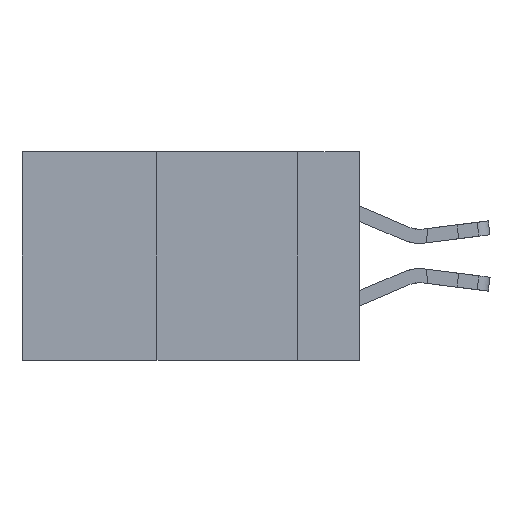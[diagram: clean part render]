
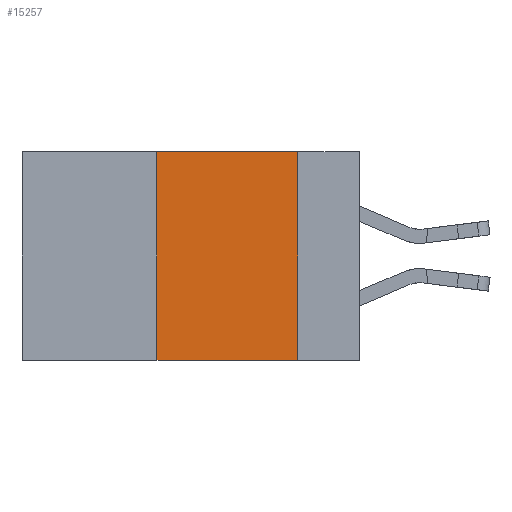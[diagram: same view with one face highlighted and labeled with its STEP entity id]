
A CAD part, left-side view. The second image highlights one B-rep face of the part: STEP entity #15257.
In plain terms, the highlighted planar face has unit normal (-1, 0, 0).
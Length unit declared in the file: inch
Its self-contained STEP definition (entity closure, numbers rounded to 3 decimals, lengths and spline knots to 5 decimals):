
#656 = DIRECTION ( 'NONE',  ( 0., 0., -1. ) ) ;
#1163 = VECTOR ( 'NONE', #656, 39.37008 ) ;
#1282 = CARTESIAN_POINT ( 'NONE',  ( 0., 0.36, 0. ) ) ;
#2127 = PLANE ( 'NONE',  #17775 ) ;
#2458 = ORIENTED_EDGE ( 'NONE', *, *, #16734, .T. ) ;
#3445 = ORIENTED_EDGE ( 'NONE', *, *, #13064, .F. ) ;
#4695 = CARTESIAN_POINT ( 'NONE',  ( 0., 0.11, -0.37 ) ) ;
#4973 = LINE ( 'NONE', #9853, #1163 ) ;
#5136 = CARTESIAN_POINT ( 'NONE',  ( 0., 0.6, 0. ) ) ;
#5137 = VERTEX_POINT ( 'NONE', #4695 ) ;
#5657 = LINE ( 'NONE', #17409, #9478 ) ;
#5901 = EDGE_CURVE ( 'NONE', #19702, #12236, #16808, .T. ) ;
#6253 = ORIENTED_EDGE ( 'NONE', *, *, #5901, .F. ) ;
#6818 = CARTESIAN_POINT ( 'NONE',  ( 0., 0.11, 0. ) ) ;
#6857 = EDGE_LOOP ( 'NONE', ( #3445, #6253, #7048, #2458 ) ) ;
#7048 = ORIENTED_EDGE ( 'NONE', *, *, #7259, .F. ) ;
#7259 = EDGE_CURVE ( 'NONE', #10920, #19702, #13660, .T. ) ;
#7915 = CARTESIAN_POINT ( 'NONE',  ( 0., 0.6, 0. ) ) ;
#9286 = CARTESIAN_POINT ( 'NONE',  ( 0., 0.36, -0.37 ) ) ;
#9478 = VECTOR ( 'NONE', #11420, 39.37008 ) ;
#9853 = CARTESIAN_POINT ( 'NONE',  ( 0., 0.11, 0. ) ) ;
#10920 = VERTEX_POINT ( 'NONE', #9286 ) ;
#11052 = VECTOR ( 'NONE', #14351, 39.37008 ) ;
#11228 = DIRECTION ( 'NONE',  ( 1., 0., 0. ) ) ;
#11420 = DIRECTION ( 'NONE',  ( 0., -1., 0. ) ) ;
#11437 = CARTESIAN_POINT ( 'NONE',  ( 0., 0.36, 0. ) ) ;
#12236 = VERTEX_POINT ( 'NONE', #6818 ) ;
#12764 = VECTOR ( 'NONE', #16914, 39.37008 ) ;
#13064 = EDGE_CURVE ( 'NONE', #12236, #5137, #4973, .T. ) ;
#13660 = LINE ( 'NONE', #11437, #11052 ) ;
#14351 = DIRECTION ( 'NONE',  ( 0., 0., 1. ) ) ;
#15257 = ADVANCED_FACE ( 'NONE', ( #16381 ), #2127, .F. ) ;
#16381 = FACE_OUTER_BOUND ( 'NONE', #6857, .T. ) ;
#16734 = EDGE_CURVE ( 'NONE', #10920, #5137, #5657, .T. ) ;
#16808 = LINE ( 'NONE', #7915, #12764 ) ;
#16914 = DIRECTION ( 'NONE',  ( 0., -1., 0. ) ) ;
#17409 = CARTESIAN_POINT ( 'NONE',  ( 0., 0.6, -0.37 ) ) ;
#17775 = AXIS2_PLACEMENT_3D ( 'NONE', #5136, #11228, #18978 ) ;
#18978 = DIRECTION ( 'NONE',  ( 0., 0., -1. ) ) ;
#19702 = VERTEX_POINT ( 'NONE', #1282 ) ;
